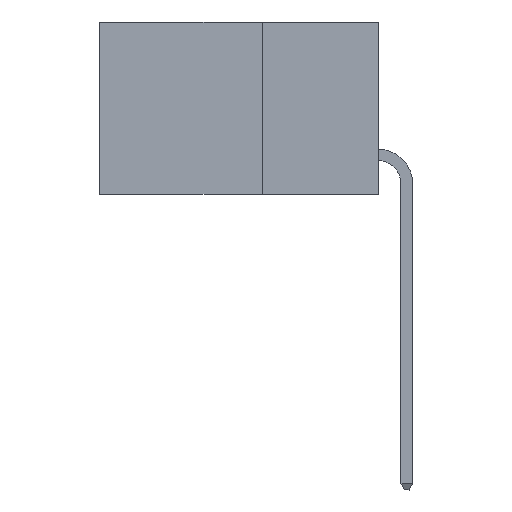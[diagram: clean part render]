
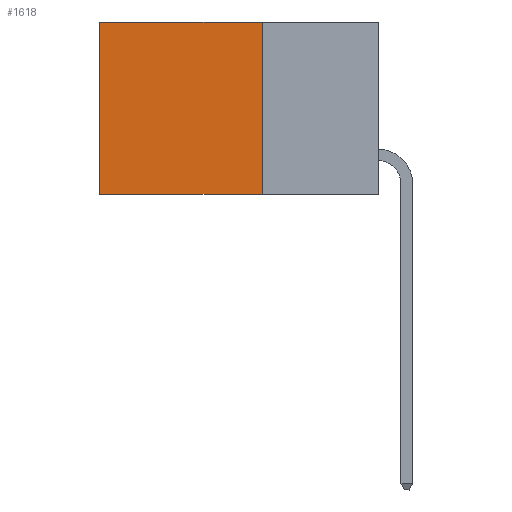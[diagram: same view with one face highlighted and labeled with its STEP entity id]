
A CAD part, left-side view. The second image highlights one B-rep face of the part: STEP entity #1618.
In plain terms, the highlighted planar face has unit normal (-1, 0, 0).
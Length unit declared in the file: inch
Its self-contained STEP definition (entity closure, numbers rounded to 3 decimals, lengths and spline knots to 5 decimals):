
#1145 = DIRECTION ( 'NONE',  ( 0., 1., 0. ) ) ;
#1618 = ADVANCED_FACE ( 'NONE', ( #2778 ), #13256, .F. ) ;
#2250 = VECTOR ( 'NONE', #22693, 39.37008 ) ;
#2778 = FACE_OUTER_BOUND ( 'NONE', #12997, .T. ) ;
#4394 = VERTEX_POINT ( 'NONE', #17132 ) ;
#5311 = CARTESIAN_POINT ( 'NONE',  ( 0.298, 0.6, 0. ) ) ;
#6521 = DIRECTION ( 'NONE',  ( 1., 0., 0. ) ) ;
#6970 = EDGE_CURVE ( 'NONE', #15103, #4394, #13958, .T. ) ;
#7109 = VERTEX_POINT ( 'NONE', #8572 ) ;
#7618 = VECTOR ( 'NONE', #1145, 39.37008 ) ;
#8413 = VECTOR ( 'NONE', #27911, 39.37008 ) ;
#8572 = CARTESIAN_POINT ( 'NONE',  ( 0.298, 0.6, -0.37 ) ) ;
#10398 = CARTESIAN_POINT ( 'NONE',  ( 0.298, 0.25, -0.37 ) ) ;
#11319 = ORIENTED_EDGE ( 'NONE', *, *, #19118, .F. ) ;
#12031 = EDGE_CURVE ( 'NONE', #16554, #7109, #25614, .T. ) ;
#12885 = DIRECTION ( 'NONE',  ( 0., 0., -1. ) ) ;
#12997 = EDGE_LOOP ( 'NONE', ( #24980, #29670, #11319, #13619 ) ) ;
#13256 = PLANE ( 'NONE',  #29698 ) ;
#13305 = CARTESIAN_POINT ( 'NONE',  ( 0.298, 0.25, -0.37 ) ) ;
#13619 = ORIENTED_EDGE ( 'NONE', *, *, #6970, .T. ) ;
#13958 = LINE ( 'NONE', #24516, #7618 ) ;
#14419 = CARTESIAN_POINT ( 'NONE',  ( 0.298, 0.25, 0. ) ) ;
#14748 = LINE ( 'NONE', #5311, #22480 ) ;
#15103 = VERTEX_POINT ( 'NONE', #14419 ) ;
#16554 = VERTEX_POINT ( 'NONE', #10398 ) ;
#17132 = CARTESIAN_POINT ( 'NONE',  ( 0.298, 0.6, 0. ) ) ;
#19118 = EDGE_CURVE ( 'NONE', #15103, #16554, #21430, .T. ) ;
#20080 = EDGE_CURVE ( 'NONE', #4394, #7109, #14748, .T. ) ;
#21430 = LINE ( 'NONE', #25422, #8413 ) ;
#22480 = VECTOR ( 'NONE', #12885, 39.37008 ) ;
#22693 = DIRECTION ( 'NONE',  ( 0., 1., 0. ) ) ;
#24516 = CARTESIAN_POINT ( 'NONE',  ( 0.298, 0.25, 0. ) ) ;
#24980 = ORIENTED_EDGE ( 'NONE', *, *, #20080, .T. ) ;
#25422 = CARTESIAN_POINT ( 'NONE',  ( 0.298, 0.25, 0. ) ) ;
#25614 = LINE ( 'NONE', #13305, #2250 ) ;
#27658 = DIRECTION ( 'NONE',  ( 0., 0., -1. ) ) ;
#27911 = DIRECTION ( 'NONE',  ( 0., 0., -1. ) ) ;
#29670 = ORIENTED_EDGE ( 'NONE', *, *, #12031, .F. ) ;
#29698 = AXIS2_PLACEMENT_3D ( 'NONE', #30247, #6521, #27658 ) ;
#30247 = CARTESIAN_POINT ( 'NONE',  ( 0.298, 0.25, 0. ) ) ;
